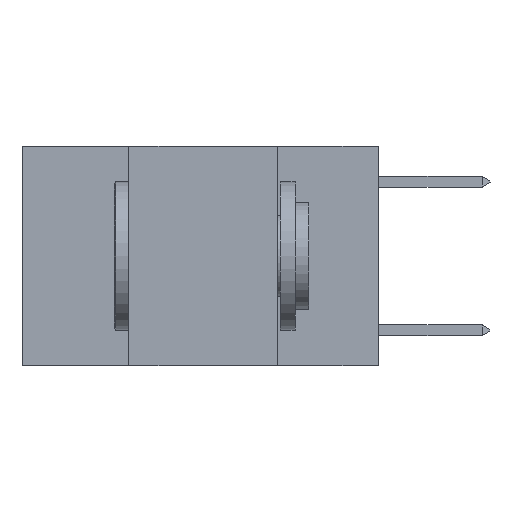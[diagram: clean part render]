
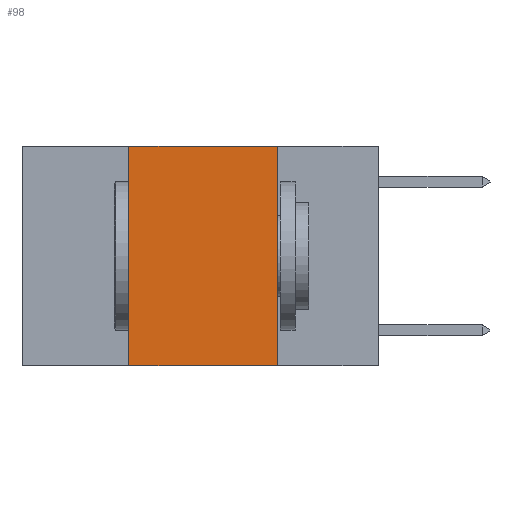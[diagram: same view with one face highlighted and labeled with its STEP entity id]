
A CAD part, left-side view. The second image highlights one B-rep face of the part: STEP entity #98.
In plain terms, the highlighted planar face has unit normal (-1, 0, 0).
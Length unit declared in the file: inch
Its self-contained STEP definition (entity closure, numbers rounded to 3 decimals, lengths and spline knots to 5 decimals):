
#98 = ADVANCED_FACE ( 'NONE', ( #3730 ), #15622, .F. ) ;
#236 = LINE ( 'NONE', #15990, #16283 ) ;
#329 = VERTEX_POINT ( 'NONE', #10532 ) ;
#793 = ORIENTED_EDGE ( 'NONE', *, *, #18137, .F. ) ;
#2040 = DIRECTION ( 'NONE',  ( 0., 0., 1. ) ) ;
#2206 = VECTOR ( 'NONE', #17331, 39.37008 ) ;
#3557 = LINE ( 'NONE', #9816, #8208 ) ;
#3730 = FACE_OUTER_BOUND ( 'NONE', #11812, .T. ) ;
#4325 = ORIENTED_EDGE ( 'NONE', *, *, #10963, .F. ) ;
#6019 = ORIENTED_EDGE ( 'NONE', *, *, #20045, .T. ) ;
#6546 = CARTESIAN_POINT ( 'NONE',  ( 0., 0.17, 0. ) ) ;
#6722 = CARTESIAN_POINT ( 'NONE',  ( 0., 0.6, -0.37 ) ) ;
#6980 = CARTESIAN_POINT ( 'NONE',  ( 0., 0.42, -0.37 ) ) ;
#7686 = CARTESIAN_POINT ( 'NONE',  ( 0., 0.17, 0. ) ) ;
#7758 = CARTESIAN_POINT ( 'NONE',  ( 0., 0.17, -0.37 ) ) ;
#8208 = VECTOR ( 'NONE', #2040, 39.37008 ) ;
#9609 = VERTEX_POINT ( 'NONE', #7686 ) ;
#9816 = CARTESIAN_POINT ( 'NONE',  ( 0., 0.42, 0. ) ) ;
#10532 = CARTESIAN_POINT ( 'NONE',  ( 0., 0.42, 0. ) ) ;
#10963 = EDGE_CURVE ( 'NONE', #9609, #17294, #18185, .T. ) ;
#11070 = EDGE_CURVE ( 'NONE', #329, #9609, #236, .T. ) ;
#11369 = DIRECTION ( 'NONE',  ( 0., -1., 0. ) ) ;
#11812 = EDGE_LOOP ( 'NONE', ( #4325, #18262, #793, #6019 ) ) ;
#14410 = LINE ( 'NONE', #6722, #17988 ) ;
#15622 = PLANE ( 'NONE',  #16723 ) ;
#15990 = CARTESIAN_POINT ( 'NONE',  ( 0., 0.6, 0. ) ) ;
#16283 = VECTOR ( 'NONE', #17524, 39.37008 ) ;
#16723 = AXIS2_PLACEMENT_3D ( 'NONE', #19144, #18572, #18274 ) ;
#17294 = VERTEX_POINT ( 'NONE', #7758 ) ;
#17331 = DIRECTION ( 'NONE',  ( 0., 0., -1. ) ) ;
#17524 = DIRECTION ( 'NONE',  ( 0., -1., 0. ) ) ;
#17988 = VECTOR ( 'NONE', #11369, 39.37008 ) ;
#18137 = EDGE_CURVE ( 'NONE', #18277, #329, #3557, .T. ) ;
#18185 = LINE ( 'NONE', #6546, #2206 ) ;
#18262 = ORIENTED_EDGE ( 'NONE', *, *, #11070, .F. ) ;
#18274 = DIRECTION ( 'NONE',  ( 0., 0., -1. ) ) ;
#18277 = VERTEX_POINT ( 'NONE', #6980 ) ;
#18572 = DIRECTION ( 'NONE',  ( 1., 0., 0. ) ) ;
#19144 = CARTESIAN_POINT ( 'NONE',  ( 0., 0.6, 0. ) ) ;
#20045 = EDGE_CURVE ( 'NONE', #18277, #17294, #14410, .T. ) ;
